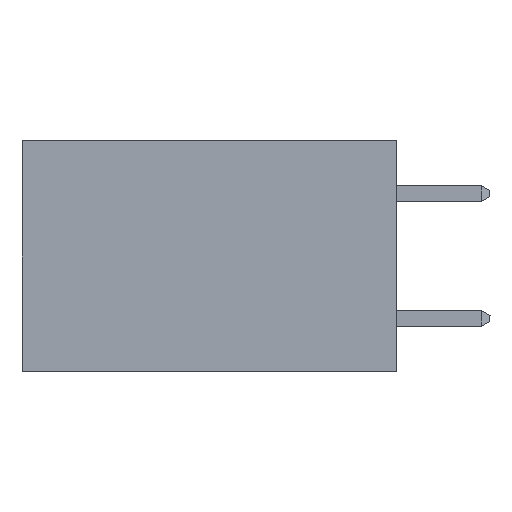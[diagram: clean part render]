
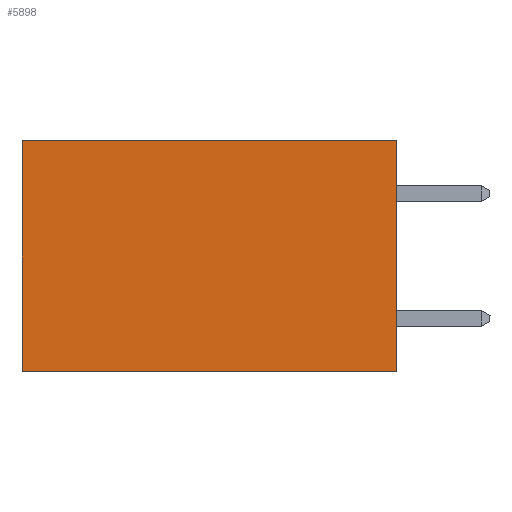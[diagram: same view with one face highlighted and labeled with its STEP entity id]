
A CAD part, left-side view. The second image highlights one B-rep face of the part: STEP entity #5898.
In plain terms, the highlighted planar face has unit normal (-1, 0, 0).
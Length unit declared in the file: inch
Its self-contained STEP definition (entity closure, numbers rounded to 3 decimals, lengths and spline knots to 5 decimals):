
#518 = CARTESIAN_POINT ( 'NONE',  ( 0.2615, 0.6, 0. ) ) ;
#590 = DIRECTION ( 'NONE',  ( 0., 1., 0. ) ) ;
#1043 = LINE ( 'NONE', #1460, #5497 ) ;
#1412 = VERTEX_POINT ( 'NONE', #11676 ) ;
#1460 = CARTESIAN_POINT ( 'NONE',  ( 0.2615, 0., 0. ) ) ;
#1969 = CARTESIAN_POINT ( 'NONE',  ( 0.2615, 0., -0.37 ) ) ;
#1998 = FACE_OUTER_BOUND ( 'NONE', #18038, .T. ) ;
#2005 = EDGE_CURVE ( 'NONE', #18041, #1412, #14434, .T. ) ;
#2045 = CARTESIAN_POINT ( 'NONE',  ( 0.2615, 0., -0.37 ) ) ;
#2329 = EDGE_CURVE ( 'NONE', #8773, #11324, #1043, .T. ) ;
#2453 = VECTOR ( 'NONE', #7243, 39.37008 ) ;
#2698 = VECTOR ( 'NONE', #590, 39.37008 ) ;
#4419 = ORIENTED_EDGE ( 'NONE', *, *, #6297, .T. ) ;
#4975 = PLANE ( 'NONE',  #7593 ) ;
#5497 = VECTOR ( 'NONE', #14442, 39.37008 ) ;
#5721 = CARTESIAN_POINT ( 'NONE',  ( 0.2615, 0., -0.37 ) ) ;
#5898 = ADVANCED_FACE ( 'NONE', ( #1998 ), #4975, .F. ) ;
#6297 = EDGE_CURVE ( 'NONE', #11324, #1412, #14195, .T. ) ;
#6469 = DIRECTION ( 'NONE',  ( 0., 0., -1. ) ) ;
#7243 = DIRECTION ( 'NONE',  ( 0., 0., -1. ) ) ;
#7593 = AXIS2_PLACEMENT_3D ( 'NONE', #1969, #15231, #6469 ) ;
#8705 = CARTESIAN_POINT ( 'NONE',  ( 0.2615, 0., 0. ) ) ;
#8773 = VERTEX_POINT ( 'NONE', #8705 ) ;
#11324 = VERTEX_POINT ( 'NONE', #518 ) ;
#11676 = CARTESIAN_POINT ( 'NONE',  ( 0.2615, 0.6, -0.37 ) ) ;
#13189 = ORIENTED_EDGE ( 'NONE', *, *, #2329, .T. ) ;
#14195 = LINE ( 'NONE', #14517, #2453 ) ;
#14433 = VECTOR ( 'NONE', #14530, 39.37008 ) ;
#14434 = LINE ( 'NONE', #2045, #2698 ) ;
#14442 = DIRECTION ( 'NONE',  ( 0., 1., 0. ) ) ;
#14509 = CARTESIAN_POINT ( 'NONE',  ( 0.2615, 0., -0.37 ) ) ;
#14517 = CARTESIAN_POINT ( 'NONE',  ( 0.2615, 0.6, -0.37 ) ) ;
#14530 = DIRECTION ( 'NONE',  ( 0., 0., -1. ) ) ;
#15231 = DIRECTION ( 'NONE',  ( 1., 0., 0. ) ) ;
#16151 = ORIENTED_EDGE ( 'NONE', *, *, #2005, .F. ) ;
#17481 = EDGE_CURVE ( 'NONE', #8773, #18041, #18349, .T. ) ;
#18038 = EDGE_LOOP ( 'NONE', ( #4419, #16151, #18522, #13189 ) ) ;
#18041 = VERTEX_POINT ( 'NONE', #14509 ) ;
#18349 = LINE ( 'NONE', #5721, #14433 ) ;
#18522 = ORIENTED_EDGE ( 'NONE', *, *, #17481, .F. ) ;
